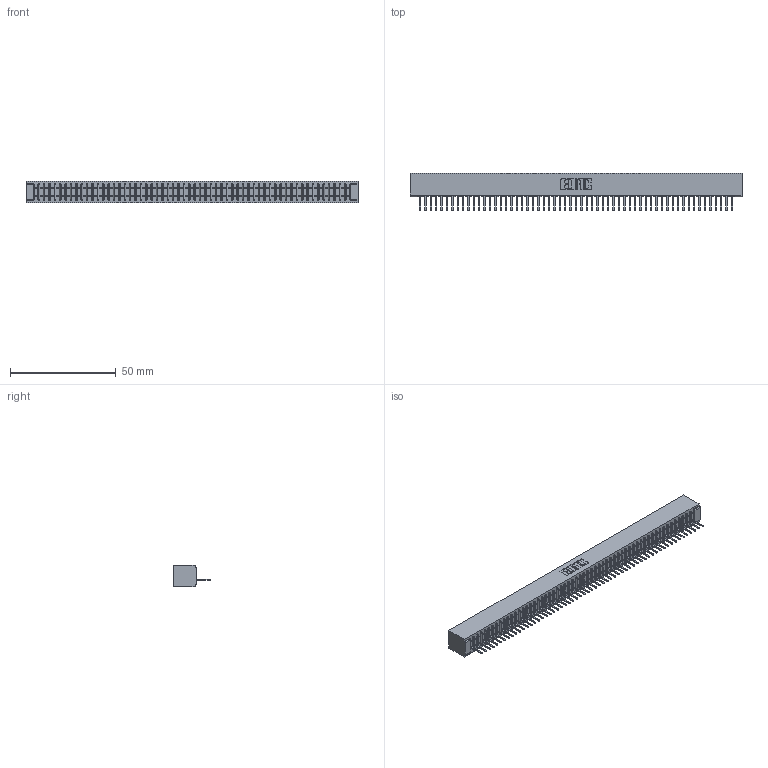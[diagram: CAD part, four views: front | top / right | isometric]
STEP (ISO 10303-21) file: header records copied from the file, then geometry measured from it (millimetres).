
FILE_DESCRIPTION (( 'STEP AP203' ), '1' );
FILE_NAME ('341-059-521-101.STEP', '2018-08-07T16:46:37', ( '' ), ( '' ), 'SwSTEP 2.0', 'SolidWorks 2016', '' );
FILE_SCHEMA (( 'CONFIG_CONTROL_DESIGN' ));
Length unit declared in the file: inch
Products named in the file (3): 341 Part_No Mounting Lugs; 341-292-001_341-292-121; 341-059-521-101
Assembly tree (60 placements, depth 2):
  341-059-521-101
    341 Part_No Mounting Lugs
    341-292-001_341-292-121  x59
Bounding box: 156.84 x 17.7 x 10.16 mm (x, y, z)
Volume: 11455.6 mm3; surface area: 18855.9 mm2
Topology: 60 solids, 60 shells, 4946 faces, 14275 edges, 9158 vertices
Faces by surface type: plane 3073, cylinder 1637, sphere 120, torus 116
Entity records: 66972 total; most frequent: CARTESIAN_POINT 11386, ORIENTED_EDGE 11374, DIRECTION 10975, EDGE_CURVE 5687, LINE 4617, VECTOR 4617, VERTEX_POINT 3590, AXIS2_PLACEMENT_3D 3179
